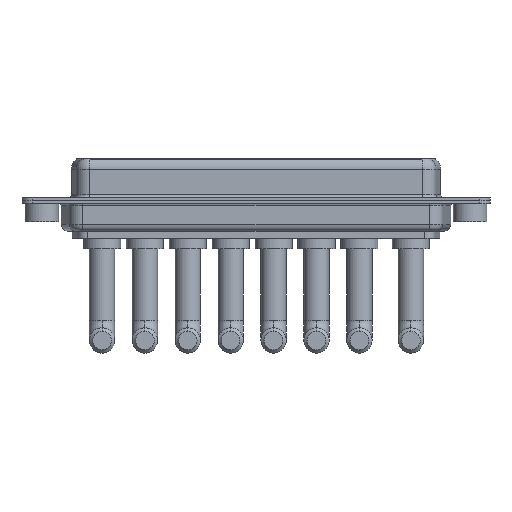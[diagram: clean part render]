
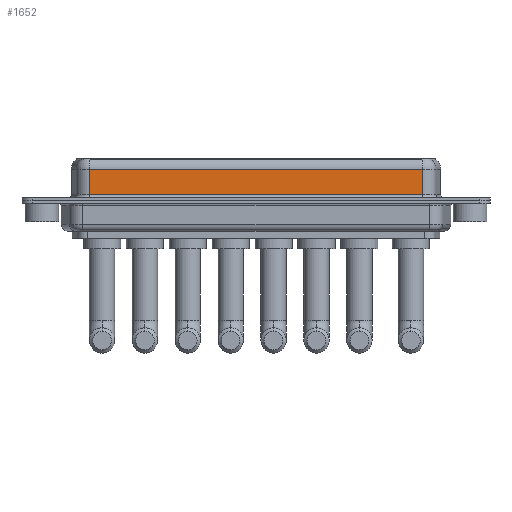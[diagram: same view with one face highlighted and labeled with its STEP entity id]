
A CAD part, front view. The second image highlights one B-rep face of the part: STEP entity #1652.
In plain terms, the highlighted planar face has unit normal (0, -1, 0).
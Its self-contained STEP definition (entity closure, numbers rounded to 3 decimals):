
#763 = EDGE_LOOP ( 'NONE', ( #4835, #6402, #7474, #4597 ) ) ;
#1197 = CARTESIAN_POINT ( 'NONE',  ( 56.462, -3.95, 4.65 ) ) ;
#1335 = PLANE ( 'NONE',  #4653 ) ;
#1338 = CARTESIAN_POINT ( 'NONE',  ( 56.462, -3.95, 4.65 ) ) ;
#1652 = ADVANCED_FACE ( 'NONE', ( #10539 ), #1335, .F. ) ;
#1922 = VERTEX_POINT ( 'NONE', #2078 ) ;
#2078 = CARTESIAN_POINT ( 'NONE',  ( 56.462, -3.95, 0.9 ) ) ;
#2173 = EDGE_CURVE ( 'NONE', #4941, #10105, #2750, .T. ) ;
#2353 = EDGE_CURVE ( 'NONE', #2997, #1922, #12490, .T. ) ;
#2430 = DIRECTION ( 'NONE',  ( 0., 1., 0. ) ) ;
#2750 = LINE ( 'NONE', #6832, #9598 ) ;
#2997 = VERTEX_POINT ( 'NONE', #1338 ) ;
#3596 = CARTESIAN_POINT ( 'NONE',  ( 7.038, -3.95, 4.65 ) ) ;
#4597 = ORIENTED_EDGE ( 'NONE', *, *, #5919, .T. ) ;
#4653 = AXIS2_PLACEMENT_3D ( 'NONE', #5450, #2430, #6520 ) ;
#4835 = ORIENTED_EDGE ( 'NONE', *, *, #2353, .F. ) ;
#4941 = VERTEX_POINT ( 'NONE', #3596 ) ;
#5186 = CARTESIAN_POINT ( 'NONE',  ( 7.038, -3.95, 0.9 ) ) ;
#5323 = VECTOR ( 'NONE', #11364, 1000. ) ;
#5450 = CARTESIAN_POINT ( 'NONE',  ( 56.462, -3.95, 6.4 ) ) ;
#5708 = DIRECTION ( 'NONE',  ( 0., 0., -1. ) ) ;
#5919 = EDGE_CURVE ( 'NONE', #10105, #1922, #7487, .T. ) ;
#5974 = VECTOR ( 'NONE', #6042, 1000. ) ;
#6042 = DIRECTION ( 'NONE',  ( -1., 0., 0. ) ) ;
#6402 = ORIENTED_EDGE ( 'NONE', *, *, #13233, .T. ) ;
#6520 = DIRECTION ( 'NONE',  ( 0., 0., 1. ) ) ;
#6832 = CARTESIAN_POINT ( 'NONE',  ( 7.038, -3.95, 6.4 ) ) ;
#7474 = ORIENTED_EDGE ( 'NONE', *, *, #2173, .T. ) ;
#7487 = LINE ( 'NONE', #10629, #13157 ) ;
#9598 = VECTOR ( 'NONE', #5708, 1000. ) ;
#10105 = VERTEX_POINT ( 'NONE', #5186 ) ;
#10330 = LINE ( 'NONE', #1197, #5974 ) ;
#10539 = FACE_OUTER_BOUND ( 'NONE', #763, .T. ) ;
#10629 = CARTESIAN_POINT ( 'NONE',  ( 56.462, -3.95, 0.9 ) ) ;
#11364 = DIRECTION ( 'NONE',  ( 0., 0., -1. ) ) ;
#11572 = DIRECTION ( 'NONE',  ( 1., 0., 0. ) ) ;
#12360 = CARTESIAN_POINT ( 'NONE',  ( 56.462, -3.95, 6.4 ) ) ;
#12490 = LINE ( 'NONE', #12360, #5323 ) ;
#13157 = VECTOR ( 'NONE', #11572, 1000. ) ;
#13233 = EDGE_CURVE ( 'NONE', #2997, #4941, #10330, .T. ) ;
